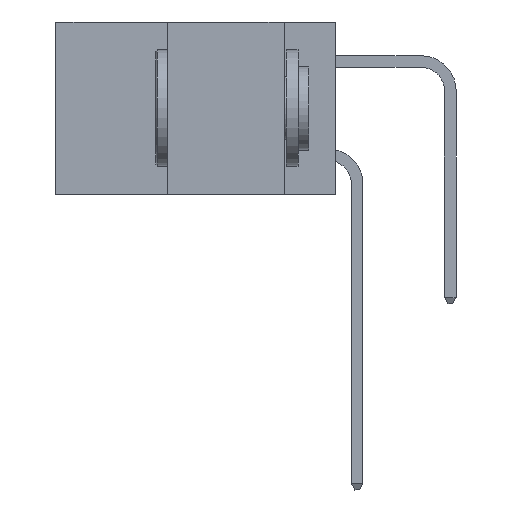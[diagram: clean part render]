
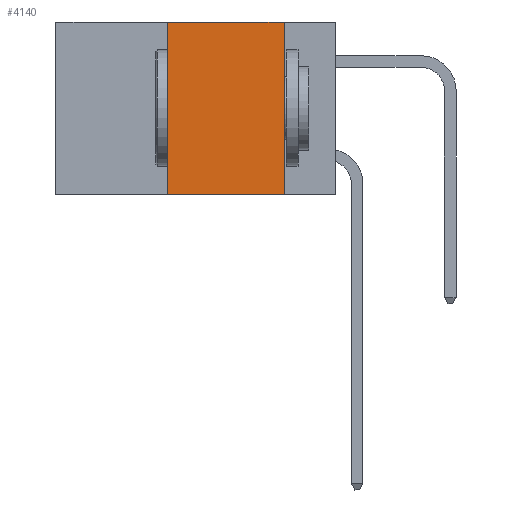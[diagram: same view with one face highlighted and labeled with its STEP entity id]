
A CAD part, left-side view. The second image highlights one B-rep face of the part: STEP entity #4140.
In plain terms, the highlighted planar face has unit normal (-1, 0, 0).
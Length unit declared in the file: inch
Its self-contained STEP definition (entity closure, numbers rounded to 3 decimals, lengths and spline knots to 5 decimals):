
#195 = CARTESIAN_POINT ( 'NONE',  ( 0., 0.36, -0.37 ) ) ;
#874 = VECTOR ( 'NONE', #3377, 39.37008 ) ;
#1057 = EDGE_CURVE ( 'NONE', #25311, #14973, #27688, .T. ) ;
#3327 = VECTOR ( 'NONE', #20956, 39.37008 ) ;
#3377 = DIRECTION ( 'NONE',  ( 0., -1., 0. ) ) ;
#4140 = ADVANCED_FACE ( 'NONE', ( #27208 ), #10764, .F. ) ;
#4225 = EDGE_LOOP ( 'NONE', ( #22101, #11676, #21261, #5761 ) ) ;
#4646 = VERTEX_POINT ( 'NONE', #6853 ) ;
#5761 = ORIENTED_EDGE ( 'NONE', *, *, #16587, .T. ) ;
#6155 = CARTESIAN_POINT ( 'NONE',  ( 0., 0.6, 0. ) ) ;
#6269 = DIRECTION ( 'NONE',  ( 1., 0., 0. ) ) ;
#6657 = LINE ( 'NONE', #10739, #874 ) ;
#6672 = LINE ( 'NONE', #6709, #16699 ) ;
#6709 = CARTESIAN_POINT ( 'NONE',  ( 0., 0.11, 0. ) ) ;
#6853 = CARTESIAN_POINT ( 'NONE',  ( 0., 0.11, -0.37 ) ) ;
#8647 = EDGE_CURVE ( 'NONE', #14973, #13771, #15448, .T. ) ;
#10739 = CARTESIAN_POINT ( 'NONE',  ( 0., 0.6, -0.37 ) ) ;
#10764 = PLANE ( 'NONE',  #25730 ) ;
#11676 = ORIENTED_EDGE ( 'NONE', *, *, #8647, .F. ) ;
#12868 = DIRECTION ( 'NONE',  ( 0., -1., 0. ) ) ;
#13771 = VERTEX_POINT ( 'NONE', #19920 ) ;
#14973 = VERTEX_POINT ( 'NONE', #15502 ) ;
#15448 = LINE ( 'NONE', #26632, #22559 ) ;
#15502 = CARTESIAN_POINT ( 'NONE',  ( 0., 0.36, 0. ) ) ;
#16587 = EDGE_CURVE ( 'NONE', #25311, #4646, #6657, .T. ) ;
#16699 = VECTOR ( 'NONE', #21060, 39.37008 ) ;
#19920 = CARTESIAN_POINT ( 'NONE',  ( 0., 0.11, 0. ) ) ;
#20000 = EDGE_CURVE ( 'NONE', #13771, #4646, #6672, .T. ) ;
#20956 = DIRECTION ( 'NONE',  ( 0., 0., 1. ) ) ;
#21060 = DIRECTION ( 'NONE',  ( 0., 0., -1. ) ) ;
#21261 = ORIENTED_EDGE ( 'NONE', *, *, #1057, .F. ) ;
#22101 = ORIENTED_EDGE ( 'NONE', *, *, #20000, .F. ) ;
#22116 = DIRECTION ( 'NONE',  ( 0., 0., -1. ) ) ;
#22559 = VECTOR ( 'NONE', #12868, 39.37008 ) ;
#25311 = VERTEX_POINT ( 'NONE', #195 ) ;
#25730 = AXIS2_PLACEMENT_3D ( 'NONE', #6155, #6269, #22116 ) ;
#26632 = CARTESIAN_POINT ( 'NONE',  ( 0., 0.6, 0. ) ) ;
#27208 = FACE_OUTER_BOUND ( 'NONE', #4225, .T. ) ;
#27688 = LINE ( 'NONE', #27808, #3327 ) ;
#27808 = CARTESIAN_POINT ( 'NONE',  ( 0., 0.36, 0. ) ) ;
